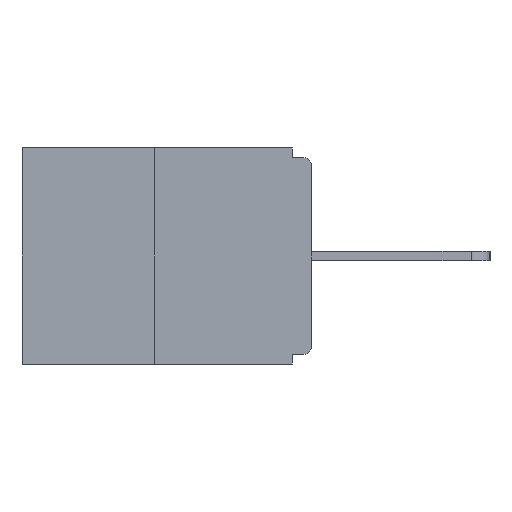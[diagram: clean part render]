
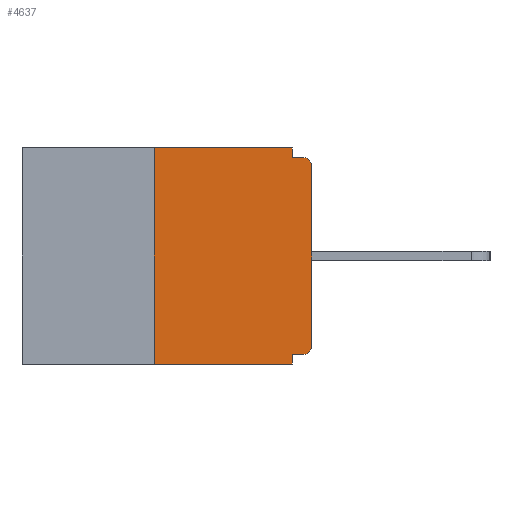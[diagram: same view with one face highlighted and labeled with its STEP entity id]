
A CAD part, left-side view. The second image highlights one B-rep face of the part: STEP entity #4637.
In plain terms, the highlighted planar face has unit normal (-1, 0, 0).
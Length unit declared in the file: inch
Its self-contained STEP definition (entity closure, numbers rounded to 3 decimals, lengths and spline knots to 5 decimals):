
#23 = DIRECTION ( 'NONE',  ( 0., 0., -1. ) ) ;
#92 = CARTESIAN_POINT ( 'NONE',  ( 0., 0., -0.015 ) ) ;
#105 = EDGE_CURVE ( 'NONE', #8333, #9948, #4040, .T. ) ;
#265 = EDGE_CURVE ( 'NONE', #10330, #7452, #8217, .T. ) ;
#445 = LINE ( 'NONE', #11595, #10269 ) ;
#676 = ORIENTED_EDGE ( 'NONE', *, *, #8067, .F. ) ;
#1520 = VECTOR ( 'NONE', #2326, 39.37008 ) ;
#1608 = DIRECTION ( 'NONE',  ( 0., 0., -1. ) ) ;
#2314 = EDGE_CURVE ( 'NONE', #4165, #5093, #3301, .T. ) ;
#2326 = DIRECTION ( 'NONE',  ( 0., -1., 0. ) ) ;
#2333 = CARTESIAN_POINT ( 'NONE',  ( 0., 0.031, 0. ) ) ;
#2807 = ORIENTED_EDGE ( 'NONE', *, *, #2314, .T. ) ;
#2976 = DIRECTION ( 'NONE',  ( 0., 0., -1. ) ) ;
#3301 = LINE ( 'NONE', #10448, #10454 ) ;
#3421 = LINE ( 'NONE', #11517, #1520 ) ;
#3559 = CARTESIAN_POINT ( 'NONE',  ( 0., 0.031, -0.343 ) ) ;
#3574 = DIRECTION ( 'NONE',  ( 0., 0., -1. ) ) ;
#3624 = EDGE_CURVE ( 'NONE', #3950, #7823, #5415, .T. ) ;
#3950 = VERTEX_POINT ( 'NONE', #7663 ) ;
#3977 = LINE ( 'NONE', #10113, #12669 ) ;
#4040 = CIRCLE ( 'NONE', #6406, 0.015 ) ;
#4052 = VERTEX_POINT ( 'NONE', #10956 ) ;
#4063 = EDGE_CURVE ( 'NONE', #3950, #10559, #8760, .T. ) ;
#4165 = VERTEX_POINT ( 'NONE', #4786 ) ;
#4637 = ADVANCED_FACE ( 'NONE', ( #7555 ), #8592, .F. ) ;
#4786 = CARTESIAN_POINT ( 'NONE',  ( 0., 0.25, -0.343 ) ) ;
#4900 = DIRECTION ( 'NONE',  ( -1., 0., 0. ) ) ;
#5043 = EDGE_CURVE ( 'NONE', #4165, #4052, #445, .T. ) ;
#5093 = VERTEX_POINT ( 'NONE', #3559 ) ;
#5356 = CARTESIAN_POINT ( 'NONE',  ( 0., 0.015, -0.015 ) ) ;
#5415 = CIRCLE ( 'NONE', #8788, 0.015 ) ;
#5657 = DIRECTION ( 'NONE',  ( 0., 0., 1. ) ) ;
#5670 = CARTESIAN_POINT ( 'NONE',  ( 0., 0.46, 0. ) ) ;
#5824 = EDGE_LOOP ( 'NONE', ( #676, #13068, #2807, #9905, #12959, #8417, #10831, #8858, #12580, #8874 ) ) ;
#6160 = CARTESIAN_POINT ( 'NONE',  ( 0., 0.031, -0.343 ) ) ;
#6406 = AXIS2_PLACEMENT_3D ( 'NONE', #8030, #4900, #6836 ) ;
#6836 = DIRECTION ( 'NONE',  ( 0., 0., -1. ) ) ;
#7096 = LINE ( 'NONE', #6160, #12208 ) ;
#7452 = VERTEX_POINT ( 'NONE', #12220 ) ;
#7540 = CARTESIAN_POINT ( 'NONE',  ( 0., 0.031, -0.328 ) ) ;
#7555 = FACE_OUTER_BOUND ( 'NONE', #5824, .T. ) ;
#7663 = CARTESIAN_POINT ( 'NONE',  ( 0., 0.015, -0.328 ) ) ;
#7671 = DIRECTION ( 'NONE',  ( 0., -1., 0. ) ) ;
#7823 = VERTEX_POINT ( 'NONE', #9231 ) ;
#7863 = EDGE_CURVE ( 'NONE', #7823, #8333, #3977, .T. ) ;
#8030 = CARTESIAN_POINT ( 'NONE',  ( 0., 0.015, -0.03 ) ) ;
#8067 = EDGE_CURVE ( 'NONE', #4052, #10330, #3421, .T. ) ;
#8131 = AXIS2_PLACEMENT_3D ( 'NONE', #5670, #11534, #3574 ) ;
#8160 = LINE ( 'NONE', #92, #12488 ) ;
#8217 = LINE ( 'NONE', #8337, #11302 ) ;
#8333 = VERTEX_POINT ( 'NONE', #11295 ) ;
#8337 = CARTESIAN_POINT ( 'NONE',  ( 0., 0.031, 0. ) ) ;
#8417 = ORIENTED_EDGE ( 'NONE', *, *, #3624, .T. ) ;
#8592 = PLANE ( 'NONE',  #8131 ) ;
#8760 = LINE ( 'NONE', #9892, #8950 ) ;
#8788 = AXIS2_PLACEMENT_3D ( 'NONE', #12617, #10790, #1608 ) ;
#8858 = ORIENTED_EDGE ( 'NONE', *, *, #105, .T. ) ;
#8874 = ORIENTED_EDGE ( 'NONE', *, *, #265, .F. ) ;
#8950 = VECTOR ( 'NONE', #12864, 39.37008 ) ;
#9231 = CARTESIAN_POINT ( 'NONE',  ( 0., 0., -0.313 ) ) ;
#9846 = EDGE_CURVE ( 'NONE', #10559, #5093, #7096, .T. ) ;
#9892 = CARTESIAN_POINT ( 'NONE',  ( 0., 0., -0.328 ) ) ;
#9905 = ORIENTED_EDGE ( 'NONE', *, *, #9846, .F. ) ;
#9948 = VERTEX_POINT ( 'NONE', #5356 ) ;
#10113 = CARTESIAN_POINT ( 'NONE',  ( 0., 0., 0. ) ) ;
#10269 = VECTOR ( 'NONE', #5657, 39.37008 ) ;
#10330 = VERTEX_POINT ( 'NONE', #2333 ) ;
#10448 = CARTESIAN_POINT ( 'NONE',  ( 0., 0.46, -0.343 ) ) ;
#10454 = VECTOR ( 'NONE', #7671, 39.37008 ) ;
#10559 = VERTEX_POINT ( 'NONE', #7540 ) ;
#10790 = DIRECTION ( 'NONE',  ( -1., 0., 0. ) ) ;
#10831 = ORIENTED_EDGE ( 'NONE', *, *, #7863, .T. ) ;
#10956 = CARTESIAN_POINT ( 'NONE',  ( 0., 0.25, 0. ) ) ;
#11295 = CARTESIAN_POINT ( 'NONE',  ( 0., 0., -0.03 ) ) ;
#11302 = VECTOR ( 'NONE', #2976, 39.37008 ) ;
#11432 = DIRECTION ( 'NONE',  ( 0., -1., 0. ) ) ;
#11517 = CARTESIAN_POINT ( 'NONE',  ( 0., 0.46, 0. ) ) ;
#11534 = DIRECTION ( 'NONE',  ( 1., 0., 0. ) ) ;
#11595 = CARTESIAN_POINT ( 'NONE',  ( 0., 0.25, 0. ) ) ;
#12208 = VECTOR ( 'NONE', #23, 39.37008 ) ;
#12220 = CARTESIAN_POINT ( 'NONE',  ( 0., 0.031, -0.015 ) ) ;
#12274 = EDGE_CURVE ( 'NONE', #7452, #9948, #8160, .T. ) ;
#12401 = DIRECTION ( 'NONE',  ( 0., 0., 1. ) ) ;
#12488 = VECTOR ( 'NONE', #11432, 39.37008 ) ;
#12580 = ORIENTED_EDGE ( 'NONE', *, *, #12274, .F. ) ;
#12617 = CARTESIAN_POINT ( 'NONE',  ( 0., 0.015, -0.313 ) ) ;
#12669 = VECTOR ( 'NONE', #12401, 39.37008 ) ;
#12864 = DIRECTION ( 'NONE',  ( 0., 1., 0. ) ) ;
#12959 = ORIENTED_EDGE ( 'NONE', *, *, #4063, .F. ) ;
#13068 = ORIENTED_EDGE ( 'NONE', *, *, #5043, .F. ) ;
